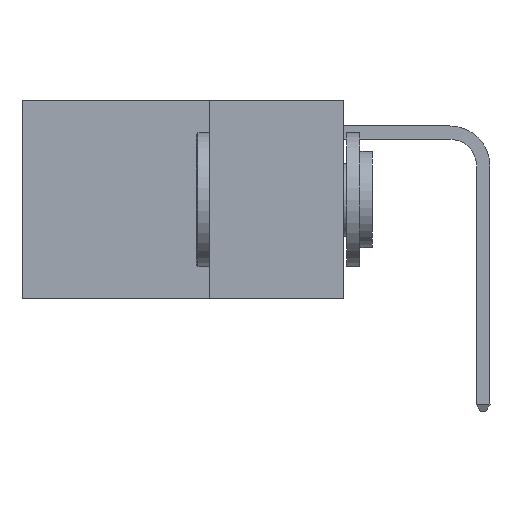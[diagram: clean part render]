
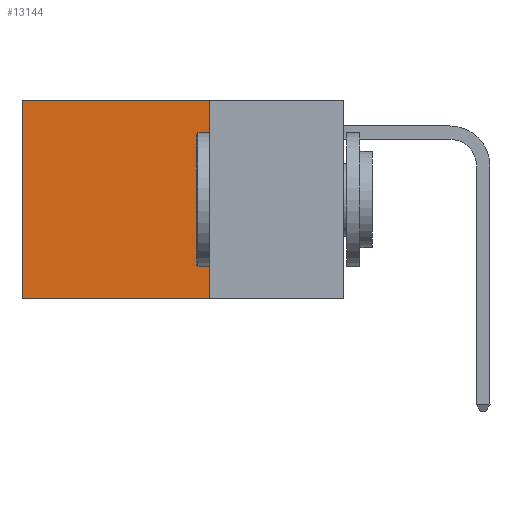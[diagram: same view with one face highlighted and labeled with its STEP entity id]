
A CAD part, left-side view. The second image highlights one B-rep face of the part: STEP entity #13144.
In plain terms, the highlighted planar face has unit normal (-1, 0, 0).
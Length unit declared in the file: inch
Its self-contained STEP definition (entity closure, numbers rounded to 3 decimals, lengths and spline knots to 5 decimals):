
#351 = EDGE_CURVE ( 'NONE', #14415, #1614, #3827, .T. ) ;
#657 = LINE ( 'NONE', #11611, #12704 ) ;
#1614 = VERTEX_POINT ( 'NONE', #18059 ) ;
#1770 = DIRECTION ( 'NONE',  ( 0., 0., -1. ) ) ;
#1849 = EDGE_CURVE ( 'NONE', #5652, #14415, #13467, .T. ) ;
#1865 = DIRECTION ( 'NONE',  ( 0., 0., -1. ) ) ;
#3151 = ORIENTED_EDGE ( 'NONE', *, *, #6315, .T. ) ;
#3545 = DIRECTION ( 'NONE',  ( 0., 1., 0. ) ) ;
#3558 = EDGE_LOOP ( 'NONE', ( #16120, #15545, #6335, #3151 ) ) ;
#3827 = LINE ( 'NONE', #15345, #5312 ) ;
#4869 = DIRECTION ( 'NONE',  ( 0., 0., -1. ) ) ;
#5312 = VECTOR ( 'NONE', #3545, 39.37008 ) ;
#5652 = VERTEX_POINT ( 'NONE', #10507 ) ;
#6273 = PLANE ( 'NONE',  #10919 ) ;
#6315 = EDGE_CURVE ( 'NONE', #5652, #7336, #12137, .T. ) ;
#6335 = ORIENTED_EDGE ( 'NONE', *, *, #1849, .F. ) ;
#7336 = VERTEX_POINT ( 'NONE', #15282 ) ;
#10390 = CARTESIAN_POINT ( 'NONE',  ( 0.2625, 0.25, 0. ) ) ;
#10507 = CARTESIAN_POINT ( 'NONE',  ( 0.2625, 0.25, 0. ) ) ;
#10829 = DIRECTION ( 'NONE',  ( 0., 1., 0. ) ) ;
#10919 = AXIS2_PLACEMENT_3D ( 'NONE', #10390, #11971, #1865 ) ;
#11611 = CARTESIAN_POINT ( 'NONE',  ( 0.2625, 0.6, 0. ) ) ;
#11684 = CARTESIAN_POINT ( 'NONE',  ( 0.2625, 0.25, 0. ) ) ;
#11971 = DIRECTION ( 'NONE',  ( 1., 0., 0. ) ) ;
#12137 = LINE ( 'NONE', #17648, #17054 ) ;
#12704 = VECTOR ( 'NONE', #4869, 39.37008 ) ;
#12717 = EDGE_CURVE ( 'NONE', #7336, #1614, #657, .T. ) ;
#12735 = VECTOR ( 'NONE', #1770, 39.37008 ) ;
#13144 = ADVANCED_FACE ( 'NONE', ( #13381 ), #6273, .F. ) ;
#13381 = FACE_OUTER_BOUND ( 'NONE', #3558, .T. ) ;
#13467 = LINE ( 'NONE', #11684, #12735 ) ;
#14415 = VERTEX_POINT ( 'NONE', #14508 ) ;
#14508 = CARTESIAN_POINT ( 'NONE',  ( 0.2625, 0.25, -0.37 ) ) ;
#15282 = CARTESIAN_POINT ( 'NONE',  ( 0.2625, 0.6, 0. ) ) ;
#15345 = CARTESIAN_POINT ( 'NONE',  ( 0.2625, 0.25, -0.37 ) ) ;
#15545 = ORIENTED_EDGE ( 'NONE', *, *, #351, .F. ) ;
#16120 = ORIENTED_EDGE ( 'NONE', *, *, #12717, .T. ) ;
#17054 = VECTOR ( 'NONE', #10829, 39.37008 ) ;
#17648 = CARTESIAN_POINT ( 'NONE',  ( 0.2625, 0.25, 0. ) ) ;
#18059 = CARTESIAN_POINT ( 'NONE',  ( 0.2625, 0.6, -0.37 ) ) ;
